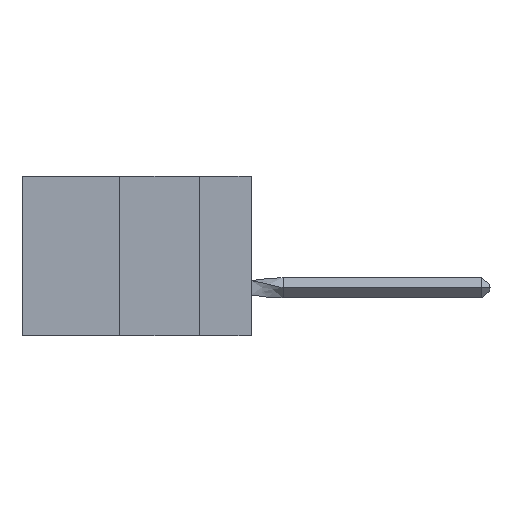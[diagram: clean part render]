
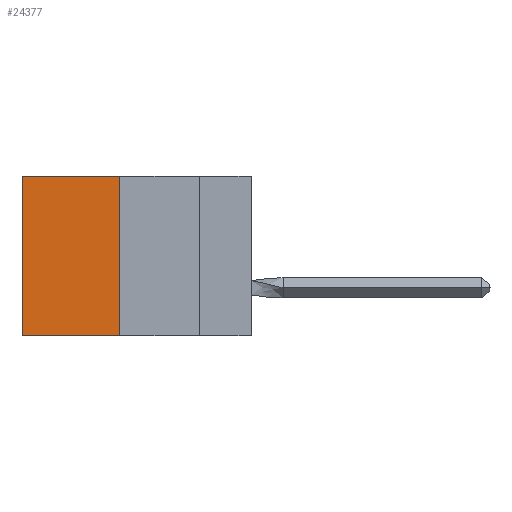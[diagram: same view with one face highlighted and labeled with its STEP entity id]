
A CAD part, left-side view. The second image highlights one B-rep face of the part: STEP entity #24377.
In plain terms, the highlighted planar face has unit normal (-1, 0, 0).
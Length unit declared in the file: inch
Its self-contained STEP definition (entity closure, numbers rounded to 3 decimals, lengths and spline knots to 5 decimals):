
#738 = FACE_OUTER_BOUND ( 'NONE', #6101, .T. ) ;
#1186 = EDGE_CURVE ( 'NONE', #3014, #23007, #17177, .T. ) ;
#1362 = CARTESIAN_POINT ( 'NONE',  ( 0.305, 0.413, -0.5 ) ) ;
#3014 = VERTEX_POINT ( 'NONE', #8050 ) ;
#4641 = ORIENTED_EDGE ( 'NONE', *, *, #1186, .T. ) ;
#4735 = AXIS2_PLACEMENT_3D ( 'NONE', #12571, #23817, #5405 ) ;
#5405 = DIRECTION ( 'NONE',  ( 0., 0., -1. ) ) ;
#6101 = EDGE_LOOP ( 'NONE', ( #4641, #12485, #18019, #23871 ) ) ;
#6413 = VECTOR ( 'NONE', #16444, 39.37008 ) ;
#6525 = DIRECTION ( 'NONE',  ( 0., 0., -1. ) ) ;
#8050 = CARTESIAN_POINT ( 'NONE',  ( 0.305, 0.72, 0. ) ) ;
#8662 = CARTESIAN_POINT ( 'NONE',  ( 0.305, 0.72, -0.5 ) ) ;
#9914 = CARTESIAN_POINT ( 'NONE',  ( 0.305, 0.72, -0.5 ) ) ;
#9930 = EDGE_CURVE ( 'NONE', #26257, #3014, #13302, .T. ) ;
#11102 = VECTOR ( 'NONE', #6525, 39.37008 ) ;
#12485 = ORIENTED_EDGE ( 'NONE', *, *, #14756, .F. ) ;
#12571 = CARTESIAN_POINT ( 'NONE',  ( 0.305, 0.413, -0.5 ) ) ;
#13302 = LINE ( 'NONE', #21263, #17485 ) ;
#14756 = EDGE_CURVE ( 'NONE', #20866, #23007, #17745, .T. ) ;
#15991 = DIRECTION ( 'NONE',  ( 0., 1., 0. ) ) ;
#16444 = DIRECTION ( 'NONE',  ( 0., 0., -1. ) ) ;
#17177 = LINE ( 'NONE', #8662, #11102 ) ;
#17485 = VECTOR ( 'NONE', #28941, 39.37008 ) ;
#17745 = LINE ( 'NONE', #1362, #21906 ) ;
#17779 = LINE ( 'NONE', #18975, #6413 ) ;
#18019 = ORIENTED_EDGE ( 'NONE', *, *, #25023, .F. ) ;
#18975 = CARTESIAN_POINT ( 'NONE',  ( 0.305, 0.413, -0.5 ) ) ;
#20866 = VERTEX_POINT ( 'NONE', #31439 ) ;
#21263 = CARTESIAN_POINT ( 'NONE',  ( 0.305, 0.413, 0. ) ) ;
#21906 = VECTOR ( 'NONE', #15991, 39.37008 ) ;
#23007 = VERTEX_POINT ( 'NONE', #9914 ) ;
#23817 = DIRECTION ( 'NONE',  ( 1., 0., 0. ) ) ;
#23871 = ORIENTED_EDGE ( 'NONE', *, *, #9930, .T. ) ;
#24377 = ADVANCED_FACE ( 'NONE', ( #738 ), #30573, .F. ) ;
#25023 = EDGE_CURVE ( 'NONE', #26257, #20866, #17779, .T. ) ;
#26257 = VERTEX_POINT ( 'NONE', #29673 ) ;
#28941 = DIRECTION ( 'NONE',  ( 0., 1., 0. ) ) ;
#29673 = CARTESIAN_POINT ( 'NONE',  ( 0.305, 0.413, 0. ) ) ;
#30573 = PLANE ( 'NONE',  #4735 ) ;
#31439 = CARTESIAN_POINT ( 'NONE',  ( 0.305, 0.413, -0.5 ) ) ;
